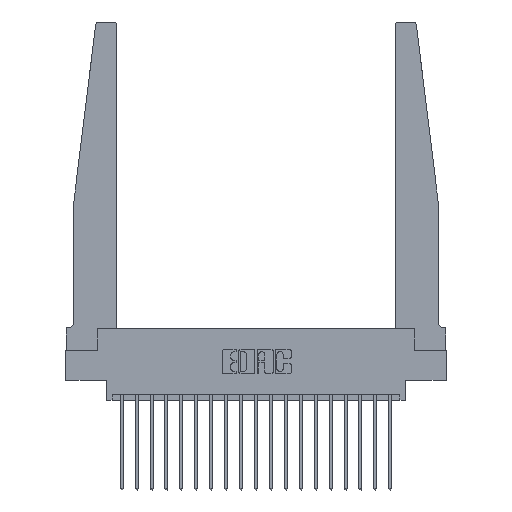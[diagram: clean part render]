
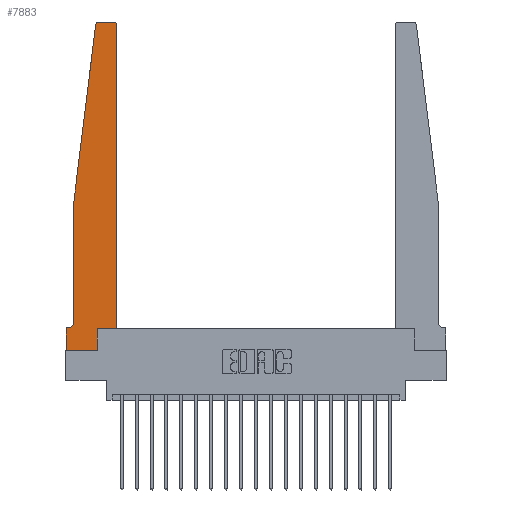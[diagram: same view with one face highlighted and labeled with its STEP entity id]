
A CAD part, top view. The second image highlights one B-rep face of the part: STEP entity #7883.
In plain terms, the highlighted planar face has unit normal (0, 0, 1).
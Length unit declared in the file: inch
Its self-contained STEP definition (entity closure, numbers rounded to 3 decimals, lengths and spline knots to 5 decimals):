
#50 = LINE ( 'NONE', #16105, #5997 ) ;
#75 = DIRECTION ( 'NONE',  ( 0., -1., 0. ) ) ;
#306 = CARTESIAN_POINT ( 'NONE',  ( 0.2605, 0.18, 0.37 ) ) ;
#575 = ORIENTED_EDGE ( 'NONE', *, *, #19532, .T. ) ;
#668 = DIRECTION ( 'NONE',  ( 0., -1., 0. ) ) ;
#705 = DIRECTION ( 'NONE',  ( 1., 0., 0. ) ) ;
#1316 = EDGE_CURVE ( 'NONE', #15665, #6807, #5088, .T. ) ;
#1480 = CARTESIAN_POINT ( 'NONE',  ( 0., 0.1875, 0.37 ) ) ;
#1756 = ORIENTED_EDGE ( 'NONE', *, *, #2646, .T. ) ;
#1905 = ORIENTED_EDGE ( 'NONE', *, *, #9803, .T. ) ;
#2158 = VERTEX_POINT ( 'NONE', #14340 ) ;
#2440 = CARTESIAN_POINT ( 'NONE',  ( 0., 0., 0.37 ) ) ;
#2646 = EDGE_CURVE ( 'NONE', #17779, #15846, #11244, .T. ) ;
#3273 = EDGE_CURVE ( 'NONE', #17692, #19840, #10551, .T. ) ;
#4015 = LINE ( 'NONE', #5810, #9033 ) ;
#4436 = DIRECTION ( 'NONE',  ( 0., 0., -1. ) ) ;
#4471 = CARTESIAN_POINT ( 'NONE',  ( 0.065, 0.2375, 0.37 ) ) ;
#4486 = ORIENTED_EDGE ( 'NONE', *, *, #17183, .T. ) ;
#4498 = AXIS2_PLACEMENT_3D ( 'NONE', #9978, #16547, #705 ) ;
#4895 = ORIENTED_EDGE ( 'NONE', *, *, #20682, .T. ) ;
#4955 = VERTEX_POINT ( 'NONE', #16631 ) ;
#5025 = DIRECTION ( 'NONE',  ( 0., 0., 1. ) ) ;
#5039 = EDGE_LOOP ( 'NONE', ( #1756, #17044, #4486, #7868, #12641, #18974, #11114, #4895, #9572, #575, #10531, #1905 ) ) ;
#5088 = LINE ( 'NONE', #8366, #14176 ) ;
#5788 = VECTOR ( 'NONE', #12724, 39.37008 ) ;
#5810 = CARTESIAN_POINT ( 'NONE',  ( 0.2605, 0.18, 0.37 ) ) ;
#5859 = VECTOR ( 'NONE', #75, 39.37008 ) ;
#5997 = VECTOR ( 'NONE', #17459, 39.37008 ) ;
#6128 = DIRECTION ( 'NONE',  ( -1., 0., 0. ) ) ;
#6222 = AXIS2_PLACEMENT_3D ( 'NONE', #19484, #5025, #11461 ) ;
#6293 = LINE ( 'NONE', #9549, #14825 ) ;
#6713 = VECTOR ( 'NONE', #668, 39.37008 ) ;
#6807 = VERTEX_POINT ( 'NONE', #12668 ) ;
#6818 = DIRECTION ( 'NONE',  ( -0.122, -0.992, 0. ) ) ;
#7868 = ORIENTED_EDGE ( 'NONE', *, *, #3273, .T. ) ;
#7883 = ADVANCED_FACE ( 'NONE', ( #9482 ), #15946, .T. ) ;
#8098 = CARTESIAN_POINT ( 'NONE',  ( 0.015, 0.1875, 0.37 ) ) ;
#8284 = CARTESIAN_POINT ( 'NONE',  ( 0.425, 0.18, 0.37 ) ) ;
#8366 = CARTESIAN_POINT ( 'NONE',  ( 0.065, 0.1875, 0.37 ) ) ;
#8687 = CARTESIAN_POINT ( 'NONE',  ( 0., 0., 0.37 ) ) ;
#8783 = DIRECTION ( 'NONE',  ( 0., 1., 0. ) ) ;
#9033 = VECTOR ( 'NONE', #8783, 39.37008 ) ;
#9245 = CIRCLE ( 'NONE', #6222, 0.03 ) ;
#9482 = FACE_OUTER_BOUND ( 'NONE', #5039, .T. ) ;
#9549 = CARTESIAN_POINT ( 'NONE',  ( 0., 0., 0.37 ) ) ;
#9572 = ORIENTED_EDGE ( 'NONE', *, *, #18001, .T. ) ;
#9803 = EDGE_CURVE ( 'NONE', #4955, #17779, #17981, .T. ) ;
#9978 = CARTESIAN_POINT ( 'NONE',  ( 0.395, 2.72, 0.37 ) ) ;
#10531 = ORIENTED_EDGE ( 'NONE', *, *, #18568, .T. ) ;
#10551 = LINE ( 'NONE', #16136, #5859 ) ;
#10747 = DIRECTION ( 'NONE',  ( 1., 0., 0. ) ) ;
#10884 = CARTESIAN_POINT ( 'NONE',  ( 0.015, 0.2375, 0.37 ) ) ;
#11114 = ORIENTED_EDGE ( 'NONE', *, *, #20132, .T. ) ;
#11244 = LINE ( 'NONE', #19267, #5788 ) ;
#11335 = LINE ( 'NONE', #8284, #16493 ) ;
#11461 = DIRECTION ( 'NONE',  ( 1., 0., 0. ) ) ;
#12210 = VERTEX_POINT ( 'NONE', #2440 ) ;
#12409 = EDGE_CURVE ( 'NONE', #15846, #17759, #9245, .T. ) ;
#12641 = ORIENTED_EDGE ( 'NONE', *, *, #13638, .T. ) ;
#12668 = CARTESIAN_POINT ( 'NONE',  ( 0., 0.1875, 0.37 ) ) ;
#12724 = DIRECTION ( 'NONE',  ( -1., 0., 0. ) ) ;
#12788 = CARTESIAN_POINT ( 'NONE',  ( 0.24675, 2.72367, 0.37 ) ) ;
#13638 = EDGE_CURVE ( 'NONE', #19840, #15665, #18366, .T. ) ;
#14068 = CARTESIAN_POINT ( 'NONE',  ( 0.395, 2.75, 0.37 ) ) ;
#14176 = VECTOR ( 'NONE', #14811, 39.37008 ) ;
#14340 = CARTESIAN_POINT ( 'NONE',  ( 0.425, 0.18, 0.37 ) ) ;
#14446 = VERTEX_POINT ( 'NONE', #20206 ) ;
#14561 = DIRECTION ( 'NONE',  ( 1., 0., 0. ) ) ;
#14743 = CARTESIAN_POINT ( 'NONE',  ( 0.065, 1.25, 0.37 ) ) ;
#14811 = DIRECTION ( 'NONE',  ( -1., 0., 0. ) ) ;
#14825 = VECTOR ( 'NONE', #10747, 39.37008 ) ;
#15375 = VERTEX_POINT ( 'NONE', #306 ) ;
#15665 = VERTEX_POINT ( 'NONE', #8098 ) ;
#15846 = VERTEX_POINT ( 'NONE', #16230 ) ;
#15946 = PLANE ( 'NONE',  #18188 ) ;
#16105 = CARTESIAN_POINT ( 'NONE',  ( 0.425, 0.18, 0.37 ) ) ;
#16136 = CARTESIAN_POINT ( 'NONE',  ( 0.065, 1.25, 0.37 ) ) ;
#16230 = CARTESIAN_POINT ( 'NONE',  ( 0.27653, 2.75, 0.37 ) ) ;
#16336 = LINE ( 'NONE', #14743, #18758 ) ;
#16493 = VECTOR ( 'NONE', #19468, 39.37008 ) ;
#16547 = DIRECTION ( 'NONE',  ( 0., 0., 1. ) ) ;
#16631 = CARTESIAN_POINT ( 'NONE',  ( 0.425, 2.72, 0.37 ) ) ;
#17044 = ORIENTED_EDGE ( 'NONE', *, *, #12409, .T. ) ;
#17183 = EDGE_CURVE ( 'NONE', #17759, #17692, #16336, .T. ) ;
#17459 = DIRECTION ( 'NONE',  ( 0., 1., 0. ) ) ;
#17685 = AXIS2_PLACEMENT_3D ( 'NONE', #10884, #4436, #6128 ) ;
#17692 = VERTEX_POINT ( 'NONE', #20087 ) ;
#17759 = VERTEX_POINT ( 'NONE', #12788 ) ;
#17779 = VERTEX_POINT ( 'NONE', #14068 ) ;
#17981 = CIRCLE ( 'NONE', #4498, 0.03 ) ;
#18001 = EDGE_CURVE ( 'NONE', #14446, #15375, #4015, .T. ) ;
#18188 = AXIS2_PLACEMENT_3D ( 'NONE', #1480, #19398, #14561 ) ;
#18366 = CIRCLE ( 'NONE', #17685, 0.05 ) ;
#18568 = EDGE_CURVE ( 'NONE', #2158, #4955, #50, .T. ) ;
#18758 = VECTOR ( 'NONE', #6818, 39.37008 ) ;
#18974 = ORIENTED_EDGE ( 'NONE', *, *, #1316, .T. ) ;
#19267 = CARTESIAN_POINT ( 'NONE',  ( 0.25, 2.75, 0.37 ) ) ;
#19398 = DIRECTION ( 'NONE',  ( 0., 0., 1. ) ) ;
#19468 = DIRECTION ( 'NONE',  ( 1., 0., 0. ) ) ;
#19484 = CARTESIAN_POINT ( 'NONE',  ( 0.27653, 2.72, 0.37 ) ) ;
#19532 = EDGE_CURVE ( 'NONE', #15375, #2158, #11335, .T. ) ;
#19840 = VERTEX_POINT ( 'NONE', #4471 ) ;
#19872 = LINE ( 'NONE', #8687, #6713 ) ;
#20087 = CARTESIAN_POINT ( 'NONE',  ( 0.065, 1.25, 0.37 ) ) ;
#20132 = EDGE_CURVE ( 'NONE', #6807, #12210, #19872, .T. ) ;
#20206 = CARTESIAN_POINT ( 'NONE',  ( 0.2605, 0., 0.37 ) ) ;
#20682 = EDGE_CURVE ( 'NONE', #12210, #14446, #6293, .T. ) ;
